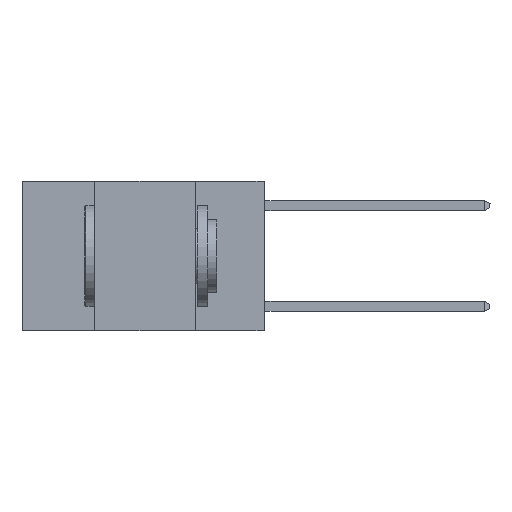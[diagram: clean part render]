
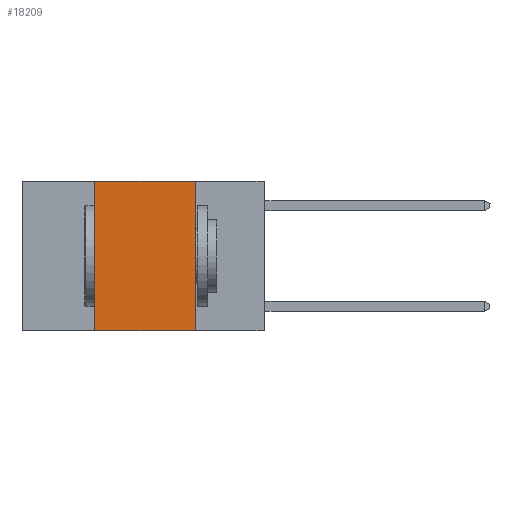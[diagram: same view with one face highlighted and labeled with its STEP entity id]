
A CAD part, left-side view. The second image highlights one B-rep face of the part: STEP entity #18209.
In plain terms, the highlighted planar face has unit normal (-1, 0, 0).
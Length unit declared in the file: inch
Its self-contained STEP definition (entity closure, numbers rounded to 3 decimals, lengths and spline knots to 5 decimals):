
#357 = DIRECTION ( 'NONE',  ( 0., 0., -1. ) ) ;
#2295 = LINE ( 'NONE', #20382, #8060 ) ;
#2468 = ORIENTED_EDGE ( 'NONE', *, *, #9975, .F. ) ;
#3183 = EDGE_CURVE ( 'NONE', #3953, #21298, #19559, .T. ) ;
#3933 = CARTESIAN_POINT ( 'NONE',  ( 0., 0.6, 0. ) ) ;
#3953 = VERTEX_POINT ( 'NONE', #19247 ) ;
#5874 = DIRECTION ( 'NONE',  ( 0., 0., 1. ) ) ;
#7736 = EDGE_CURVE ( 'NONE', #9581, #11185, #2295, .T. ) ;
#8060 = VECTOR ( 'NONE', #357, 39.37008 ) ;
#8695 = PLANE ( 'NONE',  #21375 ) ;
#9379 = ORIENTED_EDGE ( 'NONE', *, *, #3183, .F. ) ;
#9581 = VERTEX_POINT ( 'NONE', #10692 ) ;
#9975 = EDGE_CURVE ( 'NONE', #21298, #9581, #21661, .T. ) ;
#10581 = LINE ( 'NONE', #19991, #15315 ) ;
#10692 = CARTESIAN_POINT ( 'NONE',  ( 0., 0.17, 0. ) ) ;
#10903 = CARTESIAN_POINT ( 'NONE',  ( 0., 0.17, -0.37 ) ) ;
#11185 = VERTEX_POINT ( 'NONE', #10903 ) ;
#11823 = DIRECTION ( 'NONE',  ( 0., -1., 0. ) ) ;
#12440 = DIRECTION ( 'NONE',  ( 0., 0., -1. ) ) ;
#12962 = DIRECTION ( 'NONE',  ( 1., 0., 0. ) ) ;
#12967 = ORIENTED_EDGE ( 'NONE', *, *, #24429, .T. ) ;
#14286 = EDGE_LOOP ( 'NONE', ( #20935, #2468, #9379, #12967 ) ) ;
#14634 = CARTESIAN_POINT ( 'NONE',  ( 0., 0.6, 0. ) ) ;
#15315 = VECTOR ( 'NONE', #20381, 39.37008 ) ;
#17474 = CARTESIAN_POINT ( 'NONE',  ( 0., 0.42, 0. ) ) ;
#18209 = ADVANCED_FACE ( 'NONE', ( #24354 ), #8695, .F. ) ;
#19247 = CARTESIAN_POINT ( 'NONE',  ( 0., 0.42, -0.37 ) ) ;
#19559 = LINE ( 'NONE', #23606, #22216 ) ;
#19991 = CARTESIAN_POINT ( 'NONE',  ( 0., 0.6, -0.37 ) ) ;
#20381 = DIRECTION ( 'NONE',  ( 0., -1., 0. ) ) ;
#20382 = CARTESIAN_POINT ( 'NONE',  ( 0., 0.17, 0. ) ) ;
#20935 = ORIENTED_EDGE ( 'NONE', *, *, #7736, .F. ) ;
#21298 = VERTEX_POINT ( 'NONE', #17474 ) ;
#21375 = AXIS2_PLACEMENT_3D ( 'NONE', #14634, #12962, #12440 ) ;
#21661 = LINE ( 'NONE', #3933, #25077 ) ;
#22216 = VECTOR ( 'NONE', #5874, 39.37008 ) ;
#23606 = CARTESIAN_POINT ( 'NONE',  ( 0., 0.42, 0. ) ) ;
#24354 = FACE_OUTER_BOUND ( 'NONE', #14286, .T. ) ;
#24429 = EDGE_CURVE ( 'NONE', #3953, #11185, #10581, .T. ) ;
#25077 = VECTOR ( 'NONE', #11823, 39.37008 ) ;
